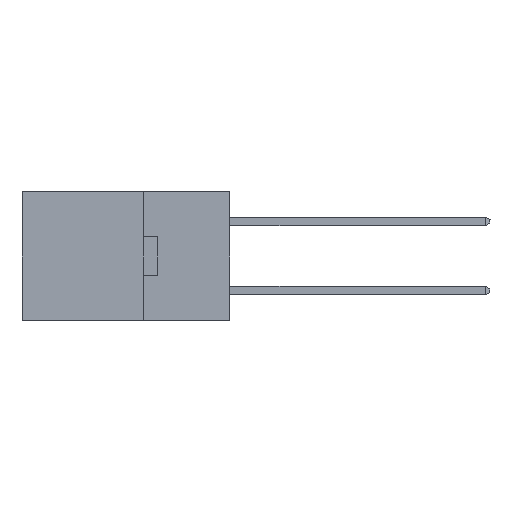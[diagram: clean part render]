
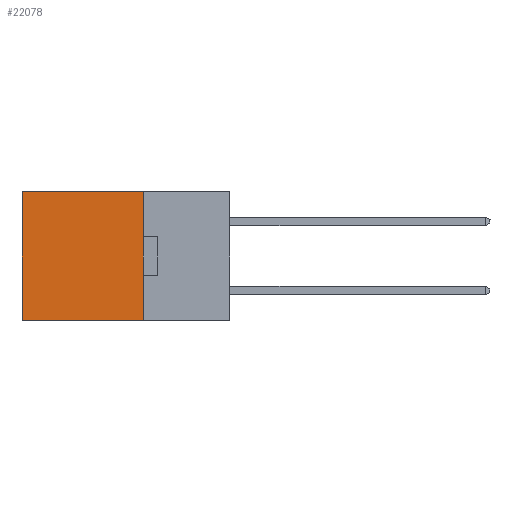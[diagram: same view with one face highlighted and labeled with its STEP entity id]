
A CAD part, left-side view. The second image highlights one B-rep face of the part: STEP entity #22078.
In plain terms, the highlighted planar face has unit normal (-1, 0, 0).
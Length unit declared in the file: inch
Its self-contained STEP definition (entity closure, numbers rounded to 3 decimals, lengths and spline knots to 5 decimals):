
#2478 = DIRECTION ( 'NONE',  ( 0., 1., 0. ) ) ;
#2771 = DIRECTION ( 'NONE',  ( 1., 0., 0. ) ) ;
#3390 = LINE ( 'NONE', #3805, #10042 ) ;
#3805 = CARTESIAN_POINT ( 'NONE',  ( 0.2615, 0.25, -0.37 ) ) ;
#4573 = LINE ( 'NONE', #21447, #10727 ) ;
#5105 = DIRECTION ( 'NONE',  ( 0., 0., -1. ) ) ;
#5727 = DIRECTION ( 'NONE',  ( 0., 0., -1. ) ) ;
#8683 = CARTESIAN_POINT ( 'NONE',  ( 0.2615, 0.25, -0.37 ) ) ;
#9024 = ORIENTED_EDGE ( 'NONE', *, *, #26226, .T. ) ;
#9668 = DIRECTION ( 'NONE',  ( 0., 0., -1. ) ) ;
#10042 = VECTOR ( 'NONE', #9668, 39.37008 ) ;
#10727 = VECTOR ( 'NONE', #2478, 39.37008 ) ;
#10987 = FACE_OUTER_BOUND ( 'NONE', #16824, .T. ) ;
#11568 = EDGE_CURVE ( 'NONE', #24244, #17372, #4573, .T. ) ;
#11664 = DIRECTION ( 'NONE',  ( 0., 1., 0. ) ) ;
#12405 = CARTESIAN_POINT ( 'NONE',  ( 0.2615, 0.25, 0. ) ) ;
#13201 = CARTESIAN_POINT ( 'NONE',  ( 0.2615, 0.6, -0.37 ) ) ;
#13821 = VERTEX_POINT ( 'NONE', #22907 ) ;
#14147 = CARTESIAN_POINT ( 'NONE',  ( 0.2615, 0.25, -0.37 ) ) ;
#15030 = EDGE_CURVE ( 'NONE', #24244, #18426, #3390, .T. ) ;
#16042 = ORIENTED_EDGE ( 'NONE', *, *, #11568, .T. ) ;
#16824 = EDGE_LOOP ( 'NONE', ( #9024, #22896, #27290, #16042 ) ) ;
#17361 = AXIS2_PLACEMENT_3D ( 'NONE', #19493, #2771, #5727 ) ;
#17372 = VERTEX_POINT ( 'NONE', #24800 ) ;
#18426 = VERTEX_POINT ( 'NONE', #8683 ) ;
#19493 = CARTESIAN_POINT ( 'NONE',  ( 0.2615, 0.25, -0.37 ) ) ;
#20298 = LINE ( 'NONE', #14147, #24114 ) ;
#21447 = CARTESIAN_POINT ( 'NONE',  ( 0.2615, 0.25, 0. ) ) ;
#21564 = LINE ( 'NONE', #13201, #26345 ) ;
#22078 = ADVANCED_FACE ( 'NONE', ( #10987 ), #23814, .F. ) ;
#22896 = ORIENTED_EDGE ( 'NONE', *, *, #26441, .F. ) ;
#22907 = CARTESIAN_POINT ( 'NONE',  ( 0.2615, 0.6, -0.37 ) ) ;
#23814 = PLANE ( 'NONE',  #17361 ) ;
#24114 = VECTOR ( 'NONE', #11664, 39.37008 ) ;
#24244 = VERTEX_POINT ( 'NONE', #12405 ) ;
#24800 = CARTESIAN_POINT ( 'NONE',  ( 0.2615, 0.6, 0. ) ) ;
#26226 = EDGE_CURVE ( 'NONE', #17372, #13821, #21564, .T. ) ;
#26345 = VECTOR ( 'NONE', #5105, 39.37008 ) ;
#26441 = EDGE_CURVE ( 'NONE', #18426, #13821, #20298, .T. ) ;
#27290 = ORIENTED_EDGE ( 'NONE', *, *, #15030, .F. ) ;
